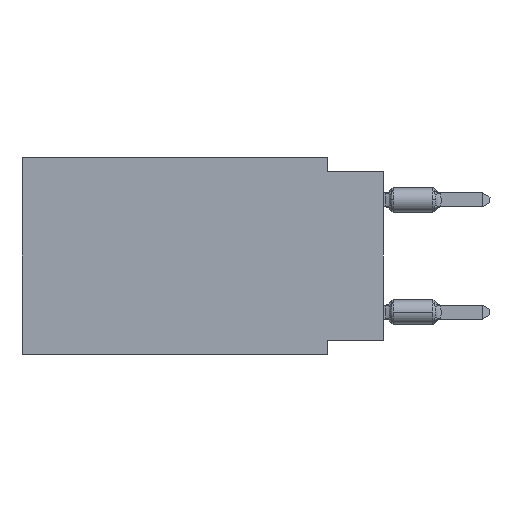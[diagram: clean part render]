
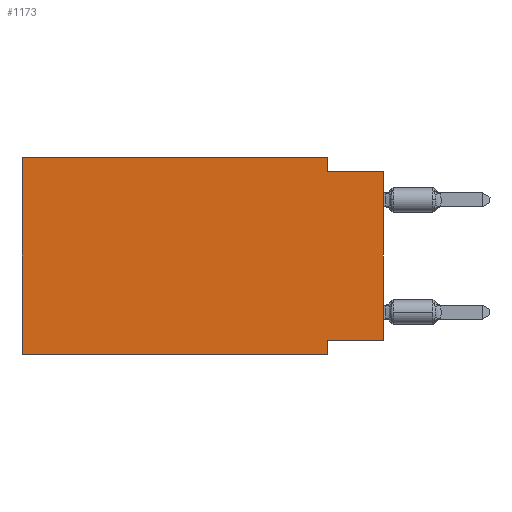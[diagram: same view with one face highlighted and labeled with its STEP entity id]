
A CAD part, left-side view. The second image highlights one B-rep face of the part: STEP entity #1173.
In plain terms, the highlighted planar face has unit normal (-1, 0, 0).
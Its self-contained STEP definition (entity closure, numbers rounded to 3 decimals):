
#120 = VERTEX_POINT ( 'NONE', #2936 ) ;
#150 = CARTESIAN_POINT ( 'NONE',  ( 0., 2.54, -8.89 ) ) ;
#956 = CARTESIAN_POINT ( 'NONE',  ( 0., 2.54, -8.255 ) ) ;
#1173 = ADVANCED_FACE ( 'NONE', ( #16994 ), #7375, .F. ) ;
#1420 = ORIENTED_EDGE ( 'NONE', *, *, #10853, .F. ) ;
#1446 = AXIS2_PLACEMENT_3D ( 'NONE', #4443, #15602, #3058 ) ;
#1770 = ORIENTED_EDGE ( 'NONE', *, *, #4909, .F. ) ;
#1824 = DIRECTION ( 'NONE',  ( 0., -1., 0. ) ) ;
#1988 = DIRECTION ( 'NONE',  ( 0., 0., -1. ) ) ;
#2390 = ORIENTED_EDGE ( 'NONE', *, *, #2460, .F. ) ;
#2406 = ORIENTED_EDGE ( 'NONE', *, *, #10599, .F. ) ;
#2430 = EDGE_CURVE ( 'NONE', #120, #8342, #4290, .T. ) ;
#2460 = EDGE_CURVE ( 'NONE', #3840, #7573, #2930, .T. ) ;
#2512 = CARTESIAN_POINT ( 'NONE',  ( 0., 0., -0.635 ) ) ;
#2930 = LINE ( 'NONE', #13995, #17552 ) ;
#2936 = CARTESIAN_POINT ( 'NONE',  ( 0., 2.54, -0.635 ) ) ;
#3058 = DIRECTION ( 'NONE',  ( 0., 0., -1. ) ) ;
#3478 = CARTESIAN_POINT ( 'NONE',  ( 0., 0., 0. ) ) ;
#3840 = VERTEX_POINT ( 'NONE', #7961 ) ;
#3939 = VECTOR ( 'NONE', #10663, 1000. ) ;
#4290 = LINE ( 'NONE', #5858, #15794 ) ;
#4343 = ORIENTED_EDGE ( 'NONE', *, *, #9670, .F. ) ;
#4371 = VERTEX_POINT ( 'NONE', #956 ) ;
#4443 = CARTESIAN_POINT ( 'NONE',  ( 0., 16.383, 0. ) ) ;
#4726 = ORIENTED_EDGE ( 'NONE', *, *, #2430, .F. ) ;
#4909 = EDGE_CURVE ( 'NONE', #11342, #4371, #16973, .T. ) ;
#4981 = CARTESIAN_POINT ( 'NONE',  ( 0., 0., -8.255 ) ) ;
#5572 = DIRECTION ( 'NONE',  ( 0., 0., -1. ) ) ;
#5858 = CARTESIAN_POINT ( 'NONE',  ( 0., 0., -0.635 ) ) ;
#6552 = CARTESIAN_POINT ( 'NONE',  ( 0., 2.54, 0. ) ) ;
#7375 = PLANE ( 'NONE',  #1446 ) ;
#7573 = VERTEX_POINT ( 'NONE', #11741 ) ;
#7576 = ORIENTED_EDGE ( 'NONE', *, *, #14652, .T. ) ;
#7961 = CARTESIAN_POINT ( 'NONE',  ( 0., 16.383, 0. ) ) ;
#8015 = CARTESIAN_POINT ( 'NONE',  ( 0., 16.383, -8.89 ) ) ;
#8342 = VERTEX_POINT ( 'NONE', #2512 ) ;
#8516 = EDGE_LOOP ( 'NONE', ( #7576, #4726, #4343, #2390, #1420, #17102, #2406, #1770 ) ) ;
#8534 = VERTEX_POINT ( 'NONE', #8751 ) ;
#8607 = DIRECTION ( 'NONE',  ( 0., -1., 0. ) ) ;
#8751 = CARTESIAN_POINT ( 'NONE',  ( 0., 16.383, -8.89 ) ) ;
#9370 = CARTESIAN_POINT ( 'NONE',  ( 0., 2.54, -8.89 ) ) ;
#9408 = DIRECTION ( 'NONE',  ( 0., 0., 1. ) ) ;
#9670 = EDGE_CURVE ( 'NONE', #7573, #120, #13513, .T. ) ;
#10599 = EDGE_CURVE ( 'NONE', #4371, #12954, #12616, .T. ) ;
#10663 = DIRECTION ( 'NONE',  ( 0., -1., 0. ) ) ;
#10853 = EDGE_CURVE ( 'NONE', #8534, #3840, #13516, .T. ) ;
#11106 = CARTESIAN_POINT ( 'NONE',  ( 0., 0., -8.255 ) ) ;
#11342 = VERTEX_POINT ( 'NONE', #4981 ) ;
#11741 = CARTESIAN_POINT ( 'NONE',  ( 0., 2.54, 0. ) ) ;
#12047 = CARTESIAN_POINT ( 'NONE',  ( 0., 16.383, 0. ) ) ;
#12565 = DIRECTION ( 'NONE',  ( 0., 1., 0. ) ) ;
#12604 = EDGE_CURVE ( 'NONE', #8534, #12954, #17818, .T. ) ;
#12616 = LINE ( 'NONE', #150, #17487 ) ;
#12954 = VERTEX_POINT ( 'NONE', #9370 ) ;
#13366 = VECTOR ( 'NONE', #1988, 1000. ) ;
#13513 = LINE ( 'NONE', #6552, #13366 ) ;
#13516 = LINE ( 'NONE', #12047, #17218 ) ;
#13995 = CARTESIAN_POINT ( 'NONE',  ( 0., 16.383, 0. ) ) ;
#14652 = EDGE_CURVE ( 'NONE', #11342, #8342, #14832, .T. ) ;
#14832 = LINE ( 'NONE', #3478, #15113 ) ;
#15008 = DIRECTION ( 'NONE',  ( 0., 0., 1. ) ) ;
#15113 = VECTOR ( 'NONE', #15008, 1000. ) ;
#15602 = DIRECTION ( 'NONE',  ( 1., 0., 0. ) ) ;
#15794 = VECTOR ( 'NONE', #1824, 1000. ) ;
#16010 = VECTOR ( 'NONE', #12565, 1000. ) ;
#16973 = LINE ( 'NONE', #11106, #16010 ) ;
#16994 = FACE_OUTER_BOUND ( 'NONE', #8516, .T. ) ;
#17102 = ORIENTED_EDGE ( 'NONE', *, *, #12604, .T. ) ;
#17218 = VECTOR ( 'NONE', #9408, 1000. ) ;
#17487 = VECTOR ( 'NONE', #5572, 1000. ) ;
#17552 = VECTOR ( 'NONE', #8607, 1000. ) ;
#17818 = LINE ( 'NONE', #8015, #3939 ) ;
